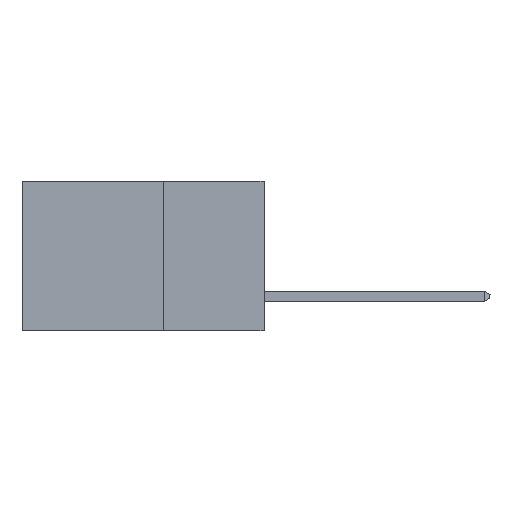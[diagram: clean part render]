
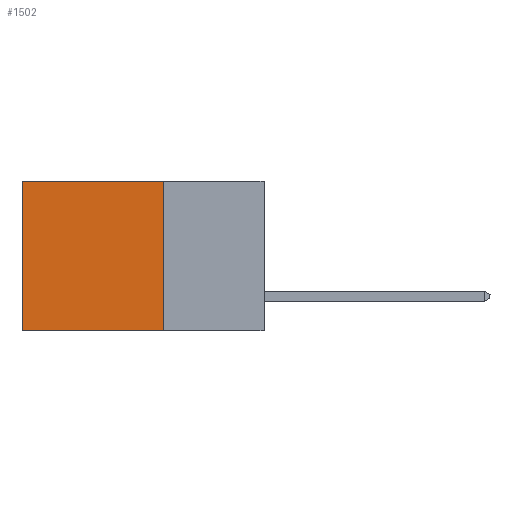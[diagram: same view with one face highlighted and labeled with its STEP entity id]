
A CAD part, left-side view. The second image highlights one B-rep face of the part: STEP entity #1502.
In plain terms, the highlighted planar face has unit normal (-1, 0, 0).
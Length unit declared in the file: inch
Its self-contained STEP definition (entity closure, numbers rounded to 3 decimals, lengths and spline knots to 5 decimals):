
#119 = CARTESIAN_POINT ( 'NONE',  ( 0.2615, 0.25, -0.37 ) ) ;
#149 = CARTESIAN_POINT ( 'NONE',  ( 0.2615, 0.25, -0.37 ) ) ;
#459 = EDGE_CURVE ( 'NONE', #1467, #9804, #6870, .T. ) ;
#611 = ORIENTED_EDGE ( 'NONE', *, *, #459, .T. ) ;
#1467 = VERTEX_POINT ( 'NONE', #14298 ) ;
#1502 = ADVANCED_FACE ( 'NONE', ( #6344 ), #6075, .F. ) ;
#1881 = EDGE_CURVE ( 'NONE', #17437, #9804, #18510, .T. ) ;
#4433 = VECTOR ( 'NONE', #6645, 39.37008 ) ;
#6075 = PLANE ( 'NONE',  #14398 ) ;
#6344 = FACE_OUTER_BOUND ( 'NONE', #9414, .T. ) ;
#6479 = DIRECTION ( 'NONE',  ( 0., 0., -1. ) ) ;
#6645 = DIRECTION ( 'NONE',  ( 0., 0., -1. ) ) ;
#6870 = LINE ( 'NONE', #24068, #23744 ) ;
#8545 = EDGE_CURVE ( 'NONE', #18553, #1467, #15138, .T. ) ;
#9414 = EDGE_LOOP ( 'NONE', ( #611, #10904, #19644, #21946 ) ) ;
#9804 = VERTEX_POINT ( 'NONE', #25606 ) ;
#10622 = VECTOR ( 'NONE', #22482, 39.37008 ) ;
#10904 = ORIENTED_EDGE ( 'NONE', *, *, #1881, .F. ) ;
#14298 = CARTESIAN_POINT ( 'NONE',  ( 0.2615, 0.6, 0. ) ) ;
#14398 = AXIS2_PLACEMENT_3D ( 'NONE', #14423, #16541, #6479 ) ;
#14423 = CARTESIAN_POINT ( 'NONE',  ( 0.2615, 0.25, -0.37 ) ) ;
#15138 = LINE ( 'NONE', #21632, #25527 ) ;
#16541 = DIRECTION ( 'NONE',  ( 1., 0., 0. ) ) ;
#16710 = LINE ( 'NONE', #24816, #4433 ) ;
#17437 = VERTEX_POINT ( 'NONE', #149 ) ;
#18510 = LINE ( 'NONE', #119, #10622 ) ;
#18553 = VERTEX_POINT ( 'NONE', #20060 ) ;
#19644 = ORIENTED_EDGE ( 'NONE', *, *, #20405, .F. ) ;
#20060 = CARTESIAN_POINT ( 'NONE',  ( 0.2615, 0.25, 0. ) ) ;
#20405 = EDGE_CURVE ( 'NONE', #18553, #17437, #16710, .T. ) ;
#21138 = DIRECTION ( 'NONE',  ( 0., 0., -1. ) ) ;
#21632 = CARTESIAN_POINT ( 'NONE',  ( 0.2615, 0.25, 0. ) ) ;
#21946 = ORIENTED_EDGE ( 'NONE', *, *, #8545, .T. ) ;
#22482 = DIRECTION ( 'NONE',  ( 0., 1., 0. ) ) ;
#23225 = DIRECTION ( 'NONE',  ( 0., 1., 0. ) ) ;
#23744 = VECTOR ( 'NONE', #21138, 39.37008 ) ;
#24068 = CARTESIAN_POINT ( 'NONE',  ( 0.2615, 0.6, -0.37 ) ) ;
#24816 = CARTESIAN_POINT ( 'NONE',  ( 0.2615, 0.25, -0.37 ) ) ;
#25527 = VECTOR ( 'NONE', #23225, 39.37008 ) ;
#25606 = CARTESIAN_POINT ( 'NONE',  ( 0.2615, 0.6, -0.37 ) ) ;
